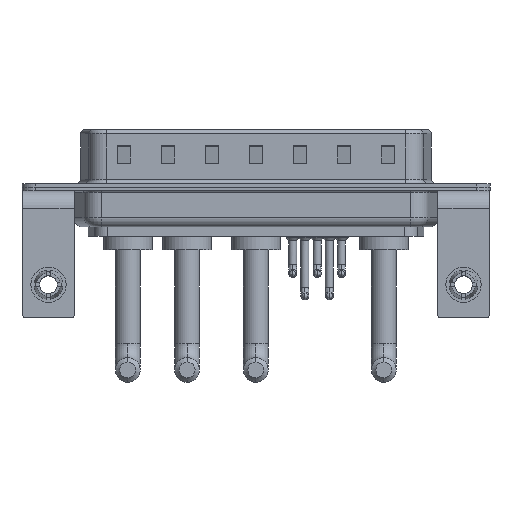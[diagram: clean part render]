
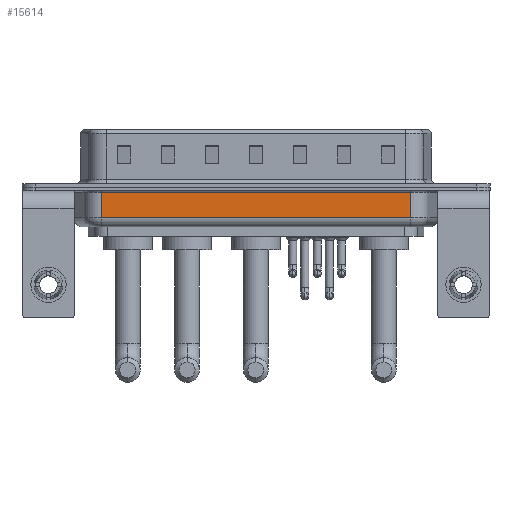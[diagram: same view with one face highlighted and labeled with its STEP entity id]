
A CAD part, front view. The second image highlights one B-rep face of the part: STEP entity #15614.
In plain terms, the highlighted planar face has unit normal (0, -1, 0).
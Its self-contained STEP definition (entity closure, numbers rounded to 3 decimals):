
#1291 = VECTOR ( 'NONE', #21556, 1000. ) ;
#1297 = CARTESIAN_POINT ( 'NONE',  ( 6.006, -5.35, -3.5 ) ) ;
#1666 = LINE ( 'NONE', #18753, #19886 ) ;
#1921 = DIRECTION ( 'NONE',  ( 0., 0., 1. ) ) ;
#3001 = CARTESIAN_POINT ( 'NONE',  ( 6.006, -5.35, -4.5 ) ) ;
#3029 = VECTOR ( 'NONE', #18323, 1000. ) ;
#3080 = LINE ( 'NONE', #1297, #18025 ) ;
#5289 = DIRECTION ( 'NONE',  ( 0., 1., 0. ) ) ;
#5799 = PLANE ( 'NONE',  #9861 ) ;
#6002 = CARTESIAN_POINT ( 'NONE',  ( 6.006, -5.35, -0.65 ) ) ;
#6367 = EDGE_CURVE ( 'NONE', #10170, #8705, #3080, .T. ) ;
#6767 = CARTESIAN_POINT ( 'NONE',  ( 6.006, -5.35, -0.65 ) ) ;
#7528 = CARTESIAN_POINT ( 'NONE',  ( 41.044, -5.35, -3.5 ) ) ;
#8705 = VERTEX_POINT ( 'NONE', #7528 ) ;
#9252 = ORIENTED_EDGE ( 'NONE', *, *, #18220, .T. ) ;
#9861 = AXIS2_PLACEMENT_3D ( 'NONE', #14965, #5289, #17102 ) ;
#10170 = VERTEX_POINT ( 'NONE', #16714 ) ;
#10603 = DIRECTION ( 'NONE',  ( 1., 0., 0. ) ) ;
#10842 = EDGE_CURVE ( 'NONE', #12014, #23190, #23194, .T. ) ;
#11561 = EDGE_LOOP ( 'NONE', ( #12594, #12930, #9252, #22044 ) ) ;
#12014 = VERTEX_POINT ( 'NONE', #15048 ) ;
#12594 = ORIENTED_EDGE ( 'NONE', *, *, #15084, .F. ) ;
#12930 = ORIENTED_EDGE ( 'NONE', *, *, #6367, .T. ) ;
#14965 = CARTESIAN_POINT ( 'NONE',  ( 6.006, -5.35, -4.5 ) ) ;
#15048 = CARTESIAN_POINT ( 'NONE',  ( 41.044, -5.35, -0.65 ) ) ;
#15084 = EDGE_CURVE ( 'NONE', #10170, #23190, #20206, .T. ) ;
#15614 = ADVANCED_FACE ( 'NONE', ( #20997 ), #5799, .F. ) ;
#16714 = CARTESIAN_POINT ( 'NONE',  ( 6.006, -5.35, -3.5 ) ) ;
#17102 = DIRECTION ( 'NONE',  ( 0., 0., 1. ) ) ;
#18025 = VECTOR ( 'NONE', #10603, 1000. ) ;
#18220 = EDGE_CURVE ( 'NONE', #8705, #12014, #1666, .T. ) ;
#18323 = DIRECTION ( 'NONE',  ( 0., 0., 1. ) ) ;
#18753 = CARTESIAN_POINT ( 'NONE',  ( 41.044, -5.35, -4.5 ) ) ;
#19886 = VECTOR ( 'NONE', #1921, 1000. ) ;
#20206 = LINE ( 'NONE', #3001, #3029 ) ;
#20997 = FACE_OUTER_BOUND ( 'NONE', #11561, .T. ) ;
#21556 = DIRECTION ( 'NONE',  ( -1., 0., 0. ) ) ;
#22044 = ORIENTED_EDGE ( 'NONE', *, *, #10842, .T. ) ;
#23190 = VERTEX_POINT ( 'NONE', #6767 ) ;
#23194 = LINE ( 'NONE', #6002, #1291 ) ;
